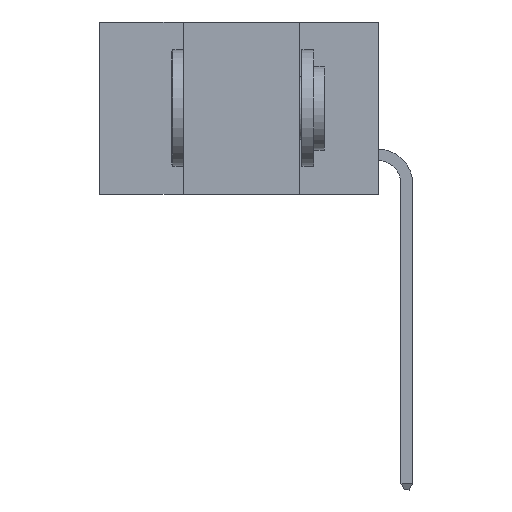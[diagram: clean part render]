
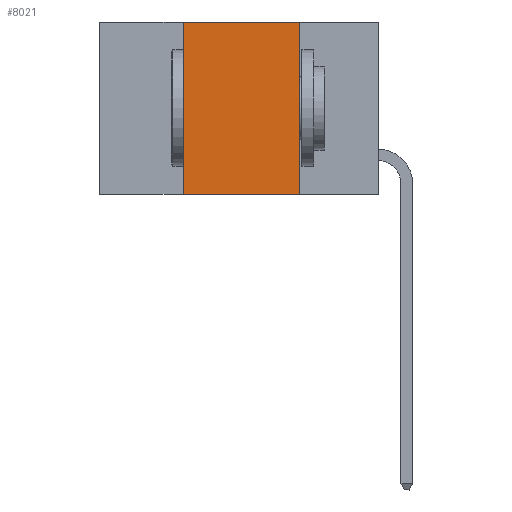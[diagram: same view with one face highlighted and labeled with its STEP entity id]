
A CAD part, left-side view. The second image highlights one B-rep face of the part: STEP entity #8021.
In plain terms, the highlighted planar face has unit normal (-1, 0, 0).
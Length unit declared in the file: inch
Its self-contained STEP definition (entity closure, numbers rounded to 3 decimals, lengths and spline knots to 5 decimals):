
#47 = VECTOR ( 'NONE', #2917, 39.37008 ) ;
#325 = CARTESIAN_POINT ( 'NONE',  ( 0., 0.42, 0. ) ) ;
#408 = CARTESIAN_POINT ( 'NONE',  ( 0., 0.6, 0. ) ) ;
#713 = LINE ( 'NONE', #4995, #11578 ) ;
#1087 = CARTESIAN_POINT ( 'NONE',  ( 0., 0.17, 0. ) ) ;
#1381 = PLANE ( 'NONE',  #5255 ) ;
#1419 = LINE ( 'NONE', #325, #4558 ) ;
#1470 = DIRECTION ( 'NONE',  ( 0., 0., -1. ) ) ;
#1659 = EDGE_CURVE ( 'NONE', #7777, #11952, #1419, .T. ) ;
#1661 = ORIENTED_EDGE ( 'NONE', *, *, #1659, .F. ) ;
#1748 = CARTESIAN_POINT ( 'NONE',  ( 0., 0.17, -0.37 ) ) ;
#2609 = VERTEX_POINT ( 'NONE', #1748 ) ;
#2917 = DIRECTION ( 'NONE',  ( 0., 0., -1. ) ) ;
#3787 = CARTESIAN_POINT ( 'NONE',  ( 0., 0.17, 0. ) ) ;
#3853 = EDGE_CURVE ( 'NONE', #4777, #2609, #9234, .T. ) ;
#4558 = VECTOR ( 'NONE', #10825, 39.37008 ) ;
#4602 = CARTESIAN_POINT ( 'NONE',  ( 0., 0.6, 0. ) ) ;
#4777 = VERTEX_POINT ( 'NONE', #3787 ) ;
#4871 = ORIENTED_EDGE ( 'NONE', *, *, #3853, .F. ) ;
#4995 = CARTESIAN_POINT ( 'NONE',  ( 0., 0.6, -0.37 ) ) ;
#5255 = AXIS2_PLACEMENT_3D ( 'NONE', #408, #9688, #1470 ) ;
#6802 = VECTOR ( 'NONE', #10906, 39.37008 ) ;
#6910 = EDGE_LOOP ( 'NONE', ( #4871, #11569, #1661, #11748 ) ) ;
#7132 = LINE ( 'NONE', #4602, #6802 ) ;
#7165 = CARTESIAN_POINT ( 'NONE',  ( 0., 0.42, 0. ) ) ;
#7777 = VERTEX_POINT ( 'NONE', #9364 ) ;
#8021 = ADVANCED_FACE ( 'NONE', ( #8343 ), #1381, .F. ) ;
#8343 = FACE_OUTER_BOUND ( 'NONE', #6910, .T. ) ;
#9234 = LINE ( 'NONE', #1087, #47 ) ;
#9364 = CARTESIAN_POINT ( 'NONE',  ( 0., 0.42, -0.37 ) ) ;
#9688 = DIRECTION ( 'NONE',  ( 1., 0., 0. ) ) ;
#10251 = EDGE_CURVE ( 'NONE', #11952, #4777, #7132, .T. ) ;
#10825 = DIRECTION ( 'NONE',  ( 0., 0., 1. ) ) ;
#10906 = DIRECTION ( 'NONE',  ( 0., -1., 0. ) ) ;
#11569 = ORIENTED_EDGE ( 'NONE', *, *, #10251, .F. ) ;
#11578 = VECTOR ( 'NONE', #13335, 39.37008 ) ;
#11748 = ORIENTED_EDGE ( 'NONE', *, *, #11900, .T. ) ;
#11900 = EDGE_CURVE ( 'NONE', #7777, #2609, #713, .T. ) ;
#11952 = VERTEX_POINT ( 'NONE', #7165 ) ;
#13335 = DIRECTION ( 'NONE',  ( 0., -1., 0. ) ) ;
